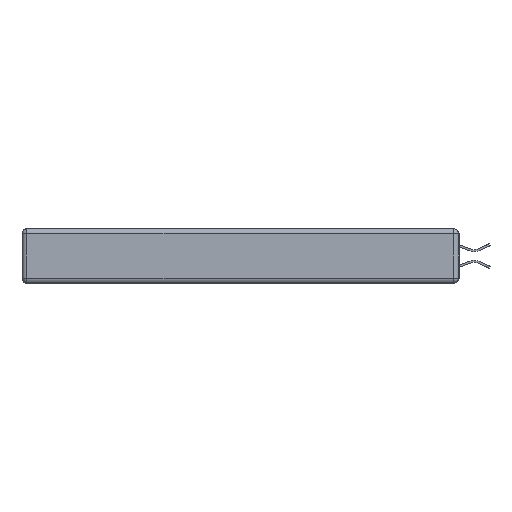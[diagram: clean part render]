
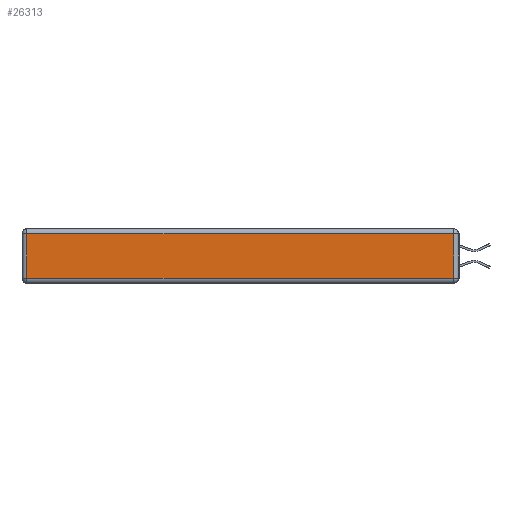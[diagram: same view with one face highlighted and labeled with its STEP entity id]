
A CAD part, left-side view. The second image highlights one B-rep face of the part: STEP entity #26313.
In plain terms, the highlighted planar face has unit normal (-1, 0, 0).
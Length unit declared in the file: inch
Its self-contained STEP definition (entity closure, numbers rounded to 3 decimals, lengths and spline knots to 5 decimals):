
#38 = LINE ( 'NONE', #17455, #29883 ) ;
#1169 = AXIS2_PLACEMENT_3D ( 'NONE', #16420, #28654, #14046 ) ;
#1511 = CARTESIAN_POINT ( 'NONE',  ( 0., 2.72, -0.313 ) ) ;
#1733 = FACE_OUTER_BOUND ( 'NONE', #21290, .T. ) ;
#1757 = CARTESIAN_POINT ( 'NONE',  ( 0., 0.03, -0.313 ) ) ;
#2812 = CARTESIAN_POINT ( 'NONE',  ( 0., 0.03, -0.343 ) ) ;
#3483 = VECTOR ( 'NONE', #27634, 39.37008 ) ;
#3496 = LINE ( 'NONE', #17222, #29069 ) ;
#4021 = VERTEX_POINT ( 'NONE', #20036 ) ;
#8019 = ORIENTED_EDGE ( 'NONE', *, *, #23337, .T. ) ;
#8591 = ORIENTED_EDGE ( 'NONE', *, *, #11658, .T. ) ;
#9188 = PLANE ( 'NONE',  #1169 ) ;
#9279 = ORIENTED_EDGE ( 'NONE', *, *, #31900, .T. ) ;
#9709 = LINE ( 'NONE', #2812, #3483 ) ;
#11658 = EDGE_CURVE ( 'NONE', #12685, #22639, #38, .T. ) ;
#12685 = VERTEX_POINT ( 'NONE', #1511 ) ;
#14046 = DIRECTION ( 'NONE',  ( 0., 0., 1. ) ) ;
#14398 = LINE ( 'NONE', #16630, #16333 ) ;
#16333 = VECTOR ( 'NONE', #21343, 39.37008 ) ;
#16420 = CARTESIAN_POINT ( 'NONE',  ( 0., 0., -0.343 ) ) ;
#16630 = CARTESIAN_POINT ( 'NONE',  ( 0., 2.75, -0.03 ) ) ;
#17222 = CARTESIAN_POINT ( 'NONE',  ( 0., 2.72, -0.343 ) ) ;
#17455 = CARTESIAN_POINT ( 'NONE',  ( 0., 0., -0.313 ) ) ;
#20036 = CARTESIAN_POINT ( 'NONE',  ( 0., 2.72, -0.03 ) ) ;
#21290 = EDGE_LOOP ( 'NONE', ( #8591, #27583, #8019, #9279 ) ) ;
#21343 = DIRECTION ( 'NONE',  ( 0., 1., 0. ) ) ;
#22639 = VERTEX_POINT ( 'NONE', #1757 ) ;
#23240 = VERTEX_POINT ( 'NONE', #23507 ) ;
#23337 = EDGE_CURVE ( 'NONE', #23240, #4021, #14398, .T. ) ;
#23507 = CARTESIAN_POINT ( 'NONE',  ( 0., 0.03, -0.03 ) ) ;
#24943 = DIRECTION ( 'NONE',  ( 0., -1., 0. ) ) ;
#26313 = ADVANCED_FACE ( 'NONE', ( #1733 ), #9188, .T. ) ;
#27583 = ORIENTED_EDGE ( 'NONE', *, *, #29669, .T. ) ;
#27634 = DIRECTION ( 'NONE',  ( 0., 0., 1. ) ) ;
#28654 = DIRECTION ( 'NONE',  ( -1., 0., 0. ) ) ;
#29069 = VECTOR ( 'NONE', #31808, 39.37008 ) ;
#29669 = EDGE_CURVE ( 'NONE', #22639, #23240, #9709, .T. ) ;
#29883 = VECTOR ( 'NONE', #24943, 39.37008 ) ;
#31808 = DIRECTION ( 'NONE',  ( 0., 0., -1. ) ) ;
#31900 = EDGE_CURVE ( 'NONE', #4021, #12685, #3496, .T. ) ;
